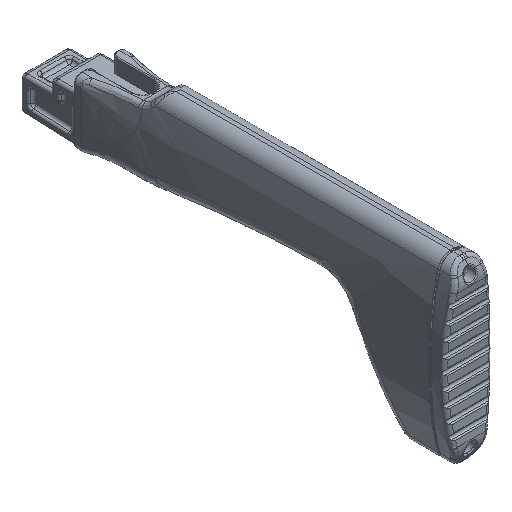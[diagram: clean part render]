
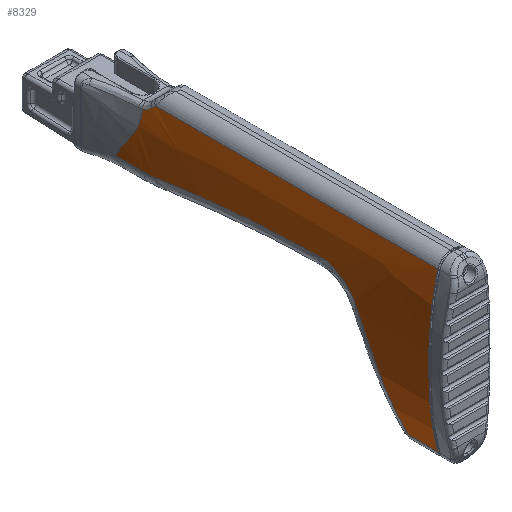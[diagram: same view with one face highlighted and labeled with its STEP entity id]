
A CAD part, isometric view. The second image highlights one B-rep face of the part: STEP entity #8329.
In plain terms, the highlighted free-form (B-spline) face has degree [1, 2] with [2, 5] control points.
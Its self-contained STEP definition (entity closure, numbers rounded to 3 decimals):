
#103=B_SPLINE_CURVE_WITH_KNOTS('',3,(#14664,#14665,#14666,#14667),
 .UNSPECIFIED.,.F.,.F.,(4,4),(-0.253,0.),.UNSPECIFIED.);
#104=B_SPLINE_CURVE_WITH_KNOTS('',3,(#14712,#14713,#14714,#14715,#14716,
#14717,#14718),.UNSPECIFIED.,.F.,.F.,(4,1,1,1,4),(-6.528,-5.596,
-4.663,-2.798,0.),.UNSPECIFIED.);
#105=B_SPLINE_CURVE_WITH_KNOTS('',3,(#14757,#14758,#14759,#14760,#14761,
#14762),.UNSPECIFIED.,.F.,.F.,(4,1,1,4),(-3.312,-2.366,
-1.419,0.),.UNSPECIFIED.);
#106=B_SPLINE_CURVE_WITH_KNOTS('',3,(#14789,#14790,#14791,#14792),
 .UNSPECIFIED.,.F.,.F.,(4,4),(-10.9,0.),.UNSPECIFIED.);
#107=B_SPLINE_CURVE_WITH_KNOTS('',3,(#14819,#14820,#14821,#14822),
 .UNSPECIFIED.,.F.,.F.,(4,4),(-0.712,0.),.UNSPECIFIED.);
#108=B_SPLINE_CURVE_WITH_KNOTS('',3,(#14847,#14848,#14849,#14850,#14851),
 .UNSPECIFIED.,.F.,.F.,(4,1,4),(23.985,24.996,26.344),
 .UNSPECIFIED.);
#109=B_SPLINE_CURVE_WITH_KNOTS('',3,(#14881,#14882,#14883,#14884,#14885,
#14886),.UNSPECIFIED.,.F.,.F.,(4,1,1,4),(0.,0.978,2.933,
3.125),.UNSPECIFIED.);
#110=B_SPLINE_CURVE_WITH_KNOTS('',3,(#14908,#14909,#14910,#14911),
 .UNSPECIFIED.,.F.,.F.,(4,4),(-0.662,-0.338),
 .UNSPECIFIED.);
#111=B_SPLINE_CURVE_WITH_KNOTS('',3,(#14912,#14913,#14914,#14915),
 .UNSPECIFIED.,.F.,.F.,(4,4),(-0.338,0.),.UNSPECIFIED.);
#126=B_SPLINE_CURVE_WITH_KNOTS('',3,(#15372,#15373,#15374,#15375,#15376,
#15377,#15378,#15379,#15380,#15381,#15382),.UNSPECIFIED.,.F.,.F.,(4,1,1,
1,1,1,1,1,4),(0.,0.763,1.525,3.05,4.575,
7.626,9.151,9.913,10.676),
 .UNSPECIFIED.);
#750=(
BOUNDED_SURFACE()
B_SPLINE_SURFACE(1,2,((#15361,#15362,#15363,#15364,#15365),(#15366,#15367,
#15368,#15369,#15370)),.UNSPECIFIED.,.F.,.F.,.F.)
B_SPLINE_SURFACE_WITH_KNOTS((2,2),(3,2,3),(0.041,3.152),
(-2.476,-1.571,-0.665),.UNSPECIFIED.)
GEOMETRIC_REPRESENTATION_ITEM()
RATIONAL_B_SPLINE_SURFACE(((1.,0.899,1.,0.899,1.),
(1.,0.899,1.,0.899,1.)))
REPRESENTATION_ITEM('')
SURFACE()
);
#1175=FACE_OUTER_BOUND('',#1752,.T.);
#1752=EDGE_LOOP('',(#6416,#6417,#6418,#6419,#6420,#6421,#6422,#6423,#6424,
#6425,#6426,#6427,#6428));
#2245=LINE('',#14825,#2596);
#2249=LINE('',#15359,#2600);
#2251=LINE('',#15383,#2602);
#2596=VECTOR('',#10558,10.);
#2600=VECTOR('',#10604,10.);
#2602=VECTOR('',#10606,10.);
#3503=VERTEX_POINT('',#13471);
#3508=VERTEX_POINT('',#13687);
#3552=VERTEX_POINT('',#14636);
#3554=VERTEX_POINT('',#14661);
#3555=VERTEX_POINT('',#14663);
#3556=VERTEX_POINT('',#14711);
#3557=VERTEX_POINT('',#14756);
#3558=VERTEX_POINT('',#14788);
#3559=VERTEX_POINT('',#14818);
#3560=VERTEX_POINT('',#14846);
#3561=VERTEX_POINT('',#14907);
#3577=VERTEX_POINT('',#15356);
#3579=VERTEX_POINT('',#15371);
#4526=EDGE_CURVE('',#3554,#3555,#103,.T.);
#4528=EDGE_CURVE('',#3552,#3556,#104,.T.);
#4530=EDGE_CURVE('',#3556,#3557,#105,.T.);
#4532=EDGE_CURVE('',#3557,#3558,#106,.T.);
#4534=EDGE_CURVE('',#3558,#3559,#107,.T.);
#4536=EDGE_CURVE('',#3559,#3503,#2245,.T.);
#4537=EDGE_CURVE('',#3503,#3560,#108,.T.);
#4539=EDGE_CURVE('',#3560,#3508,#109,.T.);
#4540=EDGE_CURVE('',#3508,#3561,#110,.T.);
#4541=EDGE_CURVE('',#3561,#3554,#111,.T.);
#4574=EDGE_CURVE('',#3552,#3577,#2249,.T.);
#4576=EDGE_CURVE('',#3579,#3577,#126,.T.);
#4577=EDGE_CURVE('',#3579,#3555,#2251,.T.);
#6416=ORIENTED_EDGE('',*,*,#4540,.F.);
#6417=ORIENTED_EDGE('',*,*,#4539,.F.);
#6418=ORIENTED_EDGE('',*,*,#4537,.F.);
#6419=ORIENTED_EDGE('',*,*,#4536,.F.);
#6420=ORIENTED_EDGE('',*,*,#4534,.F.);
#6421=ORIENTED_EDGE('',*,*,#4532,.F.);
#6422=ORIENTED_EDGE('',*,*,#4530,.F.);
#6423=ORIENTED_EDGE('',*,*,#4528,.F.);
#6424=ORIENTED_EDGE('',*,*,#4574,.T.);
#6425=ORIENTED_EDGE('',*,*,#4576,.F.);
#6426=ORIENTED_EDGE('',*,*,#4577,.T.);
#6427=ORIENTED_EDGE('',*,*,#4526,.F.);
#6428=ORIENTED_EDGE('',*,*,#4541,.F.);
#8329=ADVANCED_FACE('',(#1175),#750,.T.);
#10558=DIRECTION('',(0.,1.,0.));
#10604=DIRECTION('',(0.,-1.,0.));
#10606=DIRECTION('',(0.,1.,0.));
#13471=CARTESIAN_POINT('',(-15.76,-485.341,96.708));
#13687=CARTESIAN_POINT('',(-11.416,-499.135,128.202));
#14636=CARTESIAN_POINT('',(-10.031,-674.92,27.353));
#14661=CARTESIAN_POINT('',(-10.569,-504.818,131.424));
#14663=CARTESIAN_POINT('',(-10.031,-506.567,133.253));
#14664=CARTESIAN_POINT('Ctrl Pts',(-10.569,-504.818,
131.424));
#14665=CARTESIAN_POINT('Ctrl Pts',(-10.398,-505.402,132.033));
#14666=CARTESIAN_POINT('Ctrl Pts',(-10.219,-505.985,
132.643));
#14667=CARTESIAN_POINT('Ctrl Pts',(-10.031,-506.567,133.253));
#14711=CARTESIAN_POINT('',(-16.12,-647.054,88.811));
#14712=CARTESIAN_POINT('Ctrl Pts',(-10.031,-674.92,27.353));
#14713=CARTESIAN_POINT('Ctrl Pts',(-10.976,-673.632,
30.426));
#14714=CARTESIAN_POINT('Ctrl Pts',(-12.421,-671.02,
36.399));
#14715=CARTESIAN_POINT('Ctrl Pts',(-14.446,-665.738,
48.158));
#14716=CARTESIAN_POINT('Ctrl Pts',(-16.163,-657.746,
65.617));
#14717=CARTESIAN_POINT('Ctrl Pts',(-16.387,-651.061,80.106));
#14718=CARTESIAN_POINT('Ctrl Pts',(-16.12,-647.054,
88.811));
#14756=CARTESIAN_POINT('',(-15.023,-620.438,105.958));
#14757=CARTESIAN_POINT('Ctrl Pts',(-16.12,-647.054,
88.811));
#14758=CARTESIAN_POINT('Ctrl Pts',(-16.029,-645.699,
91.755));
#14759=CARTESIAN_POINT('Ctrl Pts',(-15.766,-642.052,97.18));
#14760=CARTESIAN_POINT('Ctrl Pts',(-15.225,-633.073,
104.094));
#14761=CARTESIAN_POINT('Ctrl Pts',(-15.016,-625.169,106.031));
#14762=CARTESIAN_POINT('Ctrl Pts',(-15.023,-620.438,
105.958));
#14788=CARTESIAN_POINT('',(-15.728,-511.831,97.222));
#14789=CARTESIAN_POINT('Ctrl Pts',(-15.023,-620.438,
105.958));
#14790=CARTESIAN_POINT('Ctrl Pts',(-15.079,-584.107,
105.394));
#14791=CARTESIAN_POINT('Ctrl Pts',(-15.399,-547.811,102.464));
#14792=CARTESIAN_POINT('Ctrl Pts',(-15.728,-511.831,
97.222));
#14818=CARTESIAN_POINT('',(-15.76,-504.734,96.708));
#14819=CARTESIAN_POINT('Ctrl Pts',(-15.728,-511.831,
97.222));
#14820=CARTESIAN_POINT('Ctrl Pts',(-15.75,-509.481,
96.88));
#14821=CARTESIAN_POINT('Ctrl Pts',(-15.76,-507.108,
96.708));
#14822=CARTESIAN_POINT('Ctrl Pts',(-15.76,-504.734,
96.708));
#14825=CARTESIAN_POINT('',(-15.76,-697.501,96.708));
#14846=CARTESIAN_POINT('',(-14.433,-494.201,111.229));
#14847=CARTESIAN_POINT('Ctrl Pts',(-15.76,-485.341,
96.708));
#14848=CARTESIAN_POINT('Ctrl Pts',(-15.626,-486.392,
98.922));
#14849=CARTESIAN_POINT('Ctrl Pts',(-15.251,-489.155,
103.977));
#14850=CARTESIAN_POINT('Ctrl Pts',(-14.754,-492.311,
108.661));
#14851=CARTESIAN_POINT('Ctrl Pts',(-14.433,-494.201,
111.229));
#14881=CARTESIAN_POINT('Ctrl Pts',(-14.433,-494.201,
111.229));
#14882=CARTESIAN_POINT('Ctrl Pts',(-14.201,-495.568,
113.087));
#14883=CARTESIAN_POINT('Ctrl Pts',(-13.407,-498.802,
118.817));
#14884=CARTESIAN_POINT('Ctrl Pts',(-12.296,-499.637,124.546));
#14885=CARTESIAN_POINT('Ctrl Pts',(-11.489,-499.184,
127.907));
#14886=CARTESIAN_POINT('Ctrl Pts',(-11.417,-499.136,
128.202));
#14907=CARTESIAN_POINT('',(-11.125,-502.153,129.36));
#14908=CARTESIAN_POINT('Ctrl Pts',(-11.416,-499.135,128.202));
#14909=CARTESIAN_POINT('Ctrl Pts',(-11.357,-500.19,128.439));
#14910=CARTESIAN_POINT('Ctrl Pts',(-11.261,-501.207,
128.835));
#14911=CARTESIAN_POINT('Ctrl Pts',(-11.125,-502.151,
129.364));
#14912=CARTESIAN_POINT('Ctrl Pts',(-11.125,-502.151,
129.364));
#14913=CARTESIAN_POINT('Ctrl Pts',(-10.984,-503.134,
129.915));
#14914=CARTESIAN_POINT('Ctrl Pts',(-10.799,-504.037,
130.611));
#14915=CARTESIAN_POINT('Ctrl Pts',(-10.569,-504.818,
131.424));
#15356=CARTESIAN_POINT('',(-10.031,-694.735,27.353));
#15359=CARTESIAN_POINT('',(-10.031,-697.501,27.353));
#15361=CARTESIAN_POINT('Ctrl Pts',(-10.031,-694.735,133.253));
#15362=CARTESIAN_POINT('Ctrl Pts',(-16.25,-694.735,
113.043));
#15363=CARTESIAN_POINT('Ctrl Pts',(-16.25,-694.735,
80.303));
#15364=CARTESIAN_POINT('Ctrl Pts',(-16.25,-694.735,
47.563));
#15365=CARTESIAN_POINT('Ctrl Pts',(-10.031,-694.735,27.353));
#15366=CARTESIAN_POINT('Ctrl Pts',(-10.031,-485.341,133.253));
#15367=CARTESIAN_POINT('Ctrl Pts',(-16.25,-485.341,
113.043));
#15368=CARTESIAN_POINT('Ctrl Pts',(-16.25,-485.341,
80.303));
#15369=CARTESIAN_POINT('Ctrl Pts',(-16.25,-485.341,
47.563));
#15370=CARTESIAN_POINT('Ctrl Pts',(-10.031,-485.341,27.353));
#15371=CARTESIAN_POINT('',(-10.031,-694.735,133.253));
#15372=CARTESIAN_POINT('Ctrl Pts',(-10.031,-694.735,133.253));
#15373=CARTESIAN_POINT('Ctrl Pts',(-10.782,-694.735,
130.811));
#15374=CARTESIAN_POINT('Ctrl Pts',(-12.045,-694.735,
125.859));
#15375=CARTESIAN_POINT('Ctrl Pts',(-13.936,-694.735,
115.844));
#15376=CARTESIAN_POINT('Ctrl Pts',(-15.446,-694.735,
103.181));
#15377=CARTESIAN_POINT('Ctrl Pts',(-16.558,-694.735,82.854));
#15378=CARTESIAN_POINT('Ctrl Pts',(-16.032,-694.735,
62.458));
#15379=CARTESIAN_POINT('Ctrl Pts',(-13.94,-694.735,
44.771));
#15380=CARTESIAN_POINT('Ctrl Pts',(-12.043,-694.735,
34.745));
#15381=CARTESIAN_POINT('Ctrl Pts',(-10.782,-694.735,
29.795));
#15382=CARTESIAN_POINT('Ctrl Pts',(-10.031,-694.735,27.353));
#15383=CARTESIAN_POINT('',(-10.031,-697.501,133.253));
